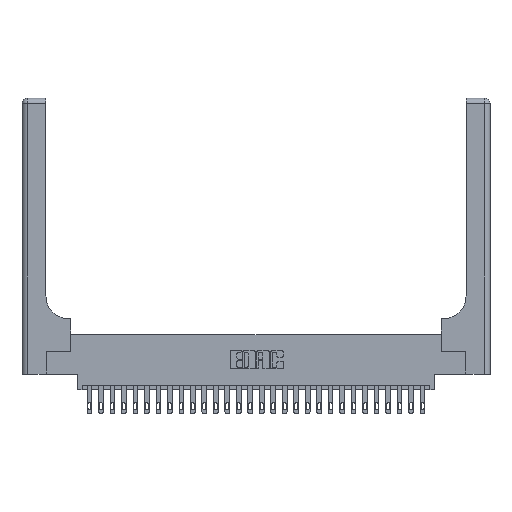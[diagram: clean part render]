
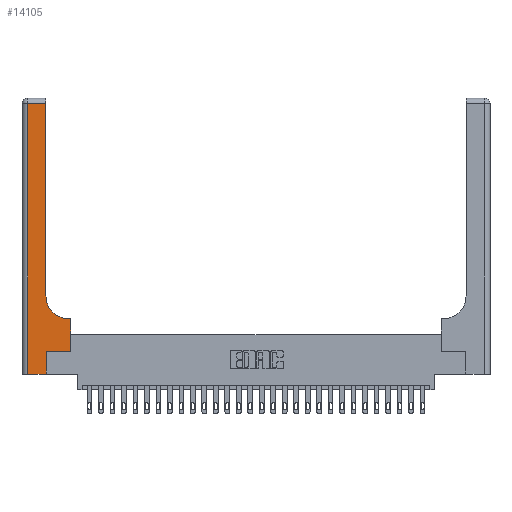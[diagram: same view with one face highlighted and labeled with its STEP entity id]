
A CAD part, top view. The second image highlights one B-rep face of the part: STEP entity #14105.
In plain terms, the highlighted planar face has unit normal (0, 0, 1).
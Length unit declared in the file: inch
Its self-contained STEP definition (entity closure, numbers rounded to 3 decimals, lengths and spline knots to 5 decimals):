
#218 = DIRECTION ( 'NONE',  ( -1., 0., 0. ) ) ;
#422 = ORIENTED_EDGE ( 'NONE', *, *, #6581, .T. ) ;
#1155 = CARTESIAN_POINT ( 'NONE',  ( 0.51, 0.85, 0.37 ) ) ;
#1413 = EDGE_CURVE ( 'NONE', #18364, #21799, #9090, .T. ) ;
#1512 = PLANE ( 'NONE',  #10462 ) ;
#2786 = CARTESIAN_POINT ( 'NONE',  ( 0.265, 0.25, 0.37 ) ) ;
#2999 = VERTEX_POINT ( 'NONE', #2786 ) ;
#3312 = VECTOR ( 'NONE', #9304, 39.37008 ) ;
#4112 = ORIENTED_EDGE ( 'NONE', *, *, #4760, .T. ) ;
#4178 = LINE ( 'NONE', #5947, #7137 ) ;
#4472 = ORIENTED_EDGE ( 'NONE', *, *, #1413, .T. ) ;
#4748 = VECTOR ( 'NONE', #8593, 39.37008 ) ;
#4760 = EDGE_CURVE ( 'NONE', #18368, #22192, #6112, .T. ) ;
#4935 = VECTOR ( 'NONE', #12982, 39.37008 ) ;
#4976 = VERTEX_POINT ( 'NONE', #20598 ) ;
#5104 = CARTESIAN_POINT ( 'NONE',  ( 0.06, 0., 0.37 ) ) ;
#5396 = VECTOR ( 'NONE', #218, 39.37008 ) ;
#5794 = LINE ( 'NONE', #24302, #16005 ) ;
#5947 = CARTESIAN_POINT ( 'NONE',  ( 0., 0., 0.37 ) ) ;
#6112 = CIRCLE ( 'NONE', #13949, 0.25 ) ;
#6581 = EDGE_CURVE ( 'NONE', #22192, #18364, #17998, .T. ) ;
#6637 = ORIENTED_EDGE ( 'NONE', *, *, #18303, .T. ) ;
#6794 = EDGE_CURVE ( 'NONE', #2999, #11624, #23945, .T. ) ;
#7137 = VECTOR ( 'NONE', #20363, 39.37008 ) ;
#8173 = ORIENTED_EDGE ( 'NONE', *, *, #20752, .T. ) ;
#8441 = VERTEX_POINT ( 'NONE', #23650 ) ;
#8593 = DIRECTION ( 'NONE',  ( 0., 1., 0. ) ) ;
#9090 = LINE ( 'NONE', #25954, #10896 ) ;
#9287 = DIRECTION ( 'NONE',  ( 0., 0., -1. ) ) ;
#9304 = DIRECTION ( 'NONE',  ( 0., 1., 0. ) ) ;
#9402 = DIRECTION ( 'NONE',  ( 1., 0., 0. ) ) ;
#9999 = EDGE_CURVE ( 'NONE', #8441, #18368, #20617, .T. ) ;
#10462 = AXIS2_PLACEMENT_3D ( 'NONE', #14039, #9287, #22186 ) ;
#10896 = VECTOR ( 'NONE', #13050, 39.37008 ) ;
#11203 = CARTESIAN_POINT ( 'NONE',  ( 0.26, 2.94, 0.37 ) ) ;
#11233 = ORIENTED_EDGE ( 'NONE', *, *, #6794, .T. ) ;
#11450 = CARTESIAN_POINT ( 'NONE',  ( 0.265, 0.25, 0.37 ) ) ;
#11624 = VERTEX_POINT ( 'NONE', #18902 ) ;
#11952 = EDGE_CURVE ( 'NONE', #21799, #14706, #5794, .T. ) ;
#12711 = EDGE_CURVE ( 'NONE', #11624, #8441, #12949, .T. ) ;
#12949 = LINE ( 'NONE', #21222, #4748 ) ;
#12982 = DIRECTION ( 'NONE',  ( 0., 1., 0. ) ) ;
#13050 = DIRECTION ( 'NONE',  ( -1., 0., 0. ) ) ;
#13484 = CARTESIAN_POINT ( 'NONE',  ( 0.06, 2.94, 0.37 ) ) ;
#13949 = AXIS2_PLACEMENT_3D ( 'NONE', #1155, #15461, #19668 ) ;
#14039 = CARTESIAN_POINT ( 'NONE',  ( 0., 3., 0.37 ) ) ;
#14105 = ADVANCED_FACE ( 'NONE', ( #17843 ), #1512, .F. ) ;
#14108 = DIRECTION ( 'NONE',  ( 0., -1., 0. ) ) ;
#14706 = VERTEX_POINT ( 'NONE', #5104 ) ;
#15461 = DIRECTION ( 'NONE',  ( 0., 0., -1. ) ) ;
#16005 = VECTOR ( 'NONE', #14108, 39.37008 ) ;
#16699 = VECTOR ( 'NONE', #9402, 39.37008 ) ;
#17305 = CARTESIAN_POINT ( 'NONE',  ( 0.265, 0., 0.37 ) ) ;
#17354 = ORIENTED_EDGE ( 'NONE', *, *, #11952, .T. ) ;
#17843 = FACE_OUTER_BOUND ( 'NONE', #19407, .T. ) ;
#17998 = LINE ( 'NONE', #26310, #3312 ) ;
#18303 = EDGE_CURVE ( 'NONE', #4976, #2999, #21377, .T. ) ;
#18364 = VERTEX_POINT ( 'NONE', #11203 ) ;
#18368 = VERTEX_POINT ( 'NONE', #20276 ) ;
#18863 = CARTESIAN_POINT ( 'NONE',  ( 0.26, 0.6, 0.37 ) ) ;
#18902 = CARTESIAN_POINT ( 'NONE',  ( 0.528, 0.25, 0.37 ) ) ;
#19157 = CARTESIAN_POINT ( 'NONE',  ( 0.26, 0.85, 0.37 ) ) ;
#19167 = ORIENTED_EDGE ( 'NONE', *, *, #12711, .T. ) ;
#19170 = ORIENTED_EDGE ( 'NONE', *, *, #9999, .T. ) ;
#19407 = EDGE_LOOP ( 'NONE', ( #422, #4472, #17354, #8173, #6637, #11233, #19167, #19170, #4112 ) ) ;
#19668 = DIRECTION ( 'NONE',  ( 1., 0., 0. ) ) ;
#20276 = CARTESIAN_POINT ( 'NONE',  ( 0.51, 0.6, 0.37 ) ) ;
#20363 = DIRECTION ( 'NONE',  ( 1., 0., 0. ) ) ;
#20598 = CARTESIAN_POINT ( 'NONE',  ( 0.265, 0., 0.37 ) ) ;
#20617 = LINE ( 'NONE', #18863, #5396 ) ;
#20752 = EDGE_CURVE ( 'NONE', #14706, #4976, #4178, .T. ) ;
#21222 = CARTESIAN_POINT ( 'NONE',  ( 0.528, 0.25, 0.37 ) ) ;
#21377 = LINE ( 'NONE', #17305, #4935 ) ;
#21799 = VERTEX_POINT ( 'NONE', #13484 ) ;
#22186 = DIRECTION ( 'NONE',  ( -1., 0., 0. ) ) ;
#22192 = VERTEX_POINT ( 'NONE', #19157 ) ;
#23650 = CARTESIAN_POINT ( 'NONE',  ( 0.528, 0.6, 0.37 ) ) ;
#23945 = LINE ( 'NONE', #11450, #16699 ) ;
#24302 = CARTESIAN_POINT ( 'NONE',  ( 0.06, 3., 0.37 ) ) ;
#25954 = CARTESIAN_POINT ( 'NONE',  ( 0., 2.94, 0.37 ) ) ;
#26310 = CARTESIAN_POINT ( 'NONE',  ( 0.26, 3., 0.37 ) ) ;
